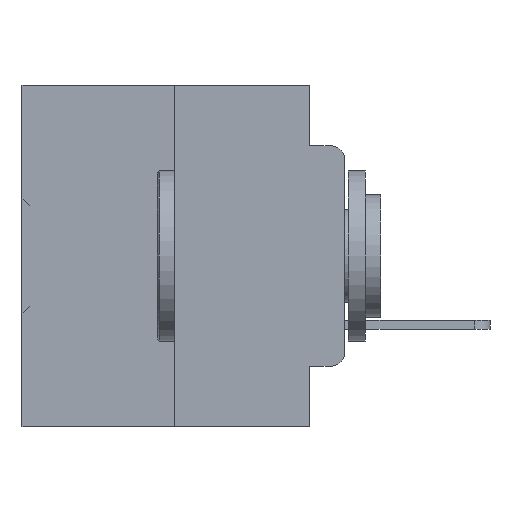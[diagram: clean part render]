
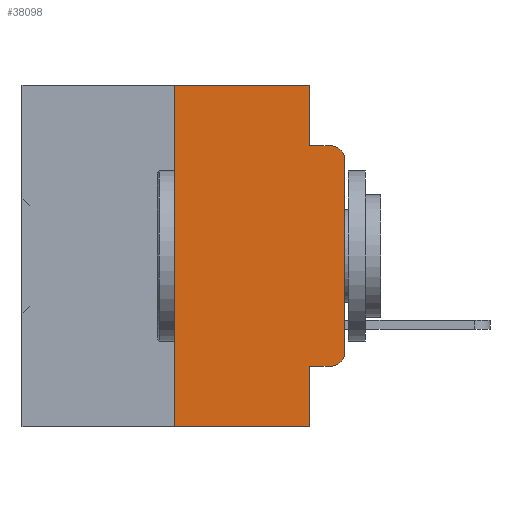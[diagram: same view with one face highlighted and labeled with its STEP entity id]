
A CAD part, left-side view. The second image highlights one B-rep face of the part: STEP entity #38098.
In plain terms, the highlighted planar face has unit normal (-1, 0, 0).
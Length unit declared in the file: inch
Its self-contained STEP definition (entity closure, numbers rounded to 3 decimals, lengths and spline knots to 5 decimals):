
#218 = ORIENTED_EDGE ( 'NONE', *, *, #24474, .T. ) ;
#294 = VERTEX_POINT ( 'NONE', #469 ) ;
#359 = EDGE_CURVE ( 'NONE', #4605, #13598, #14329, .T. ) ;
#469 = CARTESIAN_POINT ( 'NONE',  ( 0., 0.25, -0.5 ) ) ;
#636 = CARTESIAN_POINT ( 'NONE',  ( 0., 0., -0.3915 ) ) ;
#677 = DIRECTION ( 'NONE',  ( 0., 0., -1. ) ) ;
#1462 = LINE ( 'NONE', #17585, #31544 ) ;
#2384 = DIRECTION ( 'NONE',  ( 0., 0., -1. ) ) ;
#2830 = ORIENTED_EDGE ( 'NONE', *, *, #35162, .F. ) ;
#3946 = VECTOR ( 'NONE', #15467, 39.37008 ) ;
#4392 = VECTOR ( 'NONE', #37966, 39.37008 ) ;
#4605 = VERTEX_POINT ( 'NONE', #9910 ) ;
#4666 = VECTOR ( 'NONE', #22365, 39.37008 ) ;
#4873 = ORIENTED_EDGE ( 'NONE', *, *, #11984, .F. ) ;
#5578 = CARTESIAN_POINT ( 'NONE',  ( 0., 0.473, -0.5 ) ) ;
#5669 = LINE ( 'NONE', #19475, #4666 ) ;
#5768 = AXIS2_PLACEMENT_3D ( 'NONE', #32928, #18604, #38339 ) ;
#6094 = CARTESIAN_POINT ( 'NONE',  ( 0., 0.051, -0.4115 ) ) ;
#7383 = VECTOR ( 'NONE', #32266, 39.37008 ) ;
#8058 = VERTEX_POINT ( 'NONE', #17717 ) ;
#8107 = AXIS2_PLACEMENT_3D ( 'NONE', #37641, #20715, #2384 ) ;
#8116 = VECTOR ( 'NONE', #31374, 39.37008 ) ;
#8309 = CIRCLE ( 'NONE', #8107, 0.02 ) ;
#9327 = VERTEX_POINT ( 'NONE', #27889 ) ;
#9910 = CARTESIAN_POINT ( 'NONE',  ( 0., 0., -0.1085 ) ) ;
#10473 = CARTESIAN_POINT ( 'NONE',  ( 0., 0.02, -0.0885 ) ) ;
#11046 = VERTEX_POINT ( 'NONE', #13168 ) ;
#11180 = EDGE_CURVE ( 'NONE', #36608, #4605, #31614, .T. ) ;
#11320 = ORIENTED_EDGE ( 'NONE', *, *, #21795, .F. ) ;
#11788 = CARTESIAN_POINT ( 'NONE',  ( 0., 0.051, 0. ) ) ;
#11984 = EDGE_CURVE ( 'NONE', #294, #8058, #1462, .T. ) ;
#12509 = CARTESIAN_POINT ( 'NONE',  ( 0., 0.051, -0.4115 ) ) ;
#12812 = LINE ( 'NONE', #29721, #4392 ) ;
#13168 = CARTESIAN_POINT ( 'NONE',  ( 0., 0.02, -0.4115 ) ) ;
#13201 = DIRECTION ( 'NONE',  ( 0., 0., -1. ) ) ;
#13598 = VERTEX_POINT ( 'NONE', #10473 ) ;
#14329 = CIRCLE ( 'NONE', #31255, 0.02 ) ;
#15010 = EDGE_CURVE ( 'NONE', #8058, #9327, #12812, .T. ) ;
#15467 = DIRECTION ( 'NONE',  ( 0., -1., 0. ) ) ;
#16058 = ORIENTED_EDGE ( 'NONE', *, *, #35845, .F. ) ;
#17379 = ORIENTED_EDGE ( 'NONE', *, *, #11180, .T. ) ;
#17585 = CARTESIAN_POINT ( 'NONE',  ( 0., 0.25, 0. ) ) ;
#17717 = CARTESIAN_POINT ( 'NONE',  ( 0., 0.25, 0. ) ) ;
#17734 = DIRECTION ( 'NONE',  ( 0., 0., -1. ) ) ;
#18158 = CARTESIAN_POINT ( 'NONE',  ( 0., 0.02, -0.1085 ) ) ;
#18604 = DIRECTION ( 'NONE',  ( 1., 0., 0. ) ) ;
#18665 = DIRECTION ( 'NONE',  ( -1., 0., 0. ) ) ;
#19475 = CARTESIAN_POINT ( 'NONE',  ( 0., 0.051, -0.0885 ) ) ;
#20125 = CARTESIAN_POINT ( 'NONE',  ( 0., 0.051, -0.5 ) ) ;
#20182 = LINE ( 'NONE', #6094, #3946 ) ;
#20496 = DIRECTION ( 'NONE',  ( 0., 0., 1. ) ) ;
#20715 = DIRECTION ( 'NONE',  ( -1., 0., 0. ) ) ;
#21795 = EDGE_CURVE ( 'NONE', #9327, #27056, #23794, .T. ) ;
#22365 = DIRECTION ( 'NONE',  ( 0., -1., 0. ) ) ;
#22511 = EDGE_CURVE ( 'NONE', #11046, #36608, #8309, .T. ) ;
#22696 = CARTESIAN_POINT ( 'NONE',  ( 0., 0., 0. ) ) ;
#23060 = EDGE_LOOP ( 'NONE', ( #17379, #32687, #2830, #11320, #27873, #4873, #29644, #16058, #218, #25616 ) ) ;
#23794 = LINE ( 'NONE', #11788, #37811 ) ;
#24474 = EDGE_CURVE ( 'NONE', #25979, #11046, #20182, .T. ) ;
#25616 = ORIENTED_EDGE ( 'NONE', *, *, #22511, .T. ) ;
#25979 = VERTEX_POINT ( 'NONE', #12509 ) ;
#27056 = VERTEX_POINT ( 'NONE', #31674 ) ;
#27238 = FACE_OUTER_BOUND ( 'NONE', #23060, .T. ) ;
#27873 = ORIENTED_EDGE ( 'NONE', *, *, #15010, .F. ) ;
#27889 = CARTESIAN_POINT ( 'NONE',  ( 0., 0.051, 0. ) ) ;
#29644 = ORIENTED_EDGE ( 'NONE', *, *, #32544, .T. ) ;
#29721 = CARTESIAN_POINT ( 'NONE',  ( 0., 0.473, 0. ) ) ;
#31255 = AXIS2_PLACEMENT_3D ( 'NONE', #18158, #18665, #13201 ) ;
#31374 = DIRECTION ( 'NONE',  ( 0., 0., 1. ) ) ;
#31544 = VECTOR ( 'NONE', #20496, 39.37008 ) ;
#31586 = LINE ( 'NONE', #36325, #37146 ) ;
#31614 = LINE ( 'NONE', #22696, #8116 ) ;
#31674 = CARTESIAN_POINT ( 'NONE',  ( 0., 0.051, -0.0885 ) ) ;
#32266 = DIRECTION ( 'NONE',  ( 0., -1., 0. ) ) ;
#32544 = EDGE_CURVE ( 'NONE', #294, #36854, #38202, .T. ) ;
#32687 = ORIENTED_EDGE ( 'NONE', *, *, #359, .T. ) ;
#32928 = CARTESIAN_POINT ( 'NONE',  ( 0., 0.473, 0. ) ) ;
#35162 = EDGE_CURVE ( 'NONE', #27056, #13598, #5669, .T. ) ;
#35577 = PLANE ( 'NONE',  #5768 ) ;
#35845 = EDGE_CURVE ( 'NONE', #25979, #36854, #31586, .T. ) ;
#36325 = CARTESIAN_POINT ( 'NONE',  ( 0., 0.051, 0. ) ) ;
#36608 = VERTEX_POINT ( 'NONE', #636 ) ;
#36854 = VERTEX_POINT ( 'NONE', #20125 ) ;
#37146 = VECTOR ( 'NONE', #677, 39.37008 ) ;
#37641 = CARTESIAN_POINT ( 'NONE',  ( 0., 0.02, -0.3915 ) ) ;
#37811 = VECTOR ( 'NONE', #17734, 39.37008 ) ;
#37966 = DIRECTION ( 'NONE',  ( 0., -1., 0. ) ) ;
#38098 = ADVANCED_FACE ( 'NONE', ( #27238 ), #35577, .F. ) ;
#38202 = LINE ( 'NONE', #5578, #7383 ) ;
#38339 = DIRECTION ( 'NONE',  ( 0., 0., -1. ) ) ;
